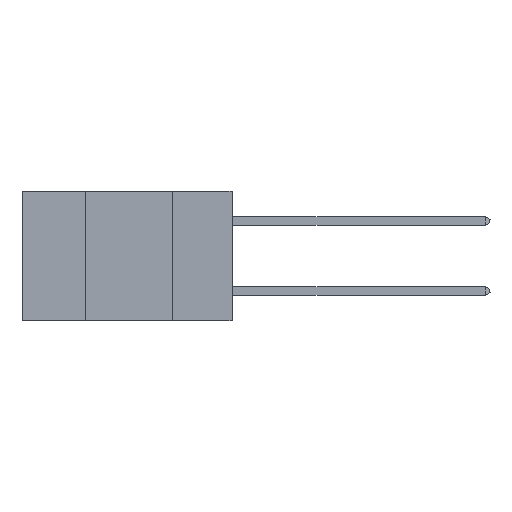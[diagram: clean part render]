
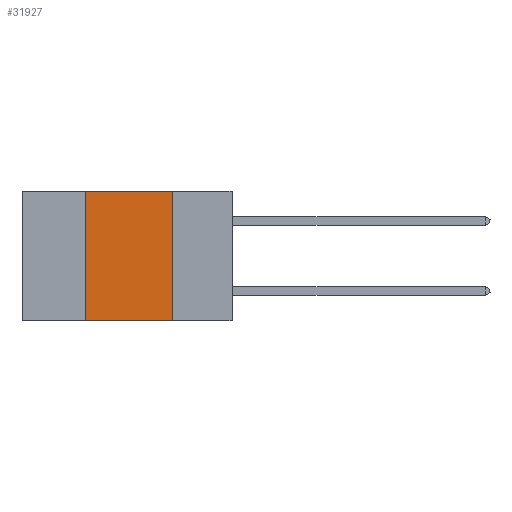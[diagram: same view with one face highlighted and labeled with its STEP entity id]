
A CAD part, left-side view. The second image highlights one B-rep face of the part: STEP entity #31927.
In plain terms, the highlighted planar face has unit normal (-1, 0, 0).
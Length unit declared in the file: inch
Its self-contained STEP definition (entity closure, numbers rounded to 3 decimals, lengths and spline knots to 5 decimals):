
#626 = LINE ( 'NONE', #4560, #36915 ) ;
#800 = VERTEX_POINT ( 'NONE', #27036 ) ;
#1800 = CARTESIAN_POINT ( 'NONE',  ( 0., 0.6, -0.37 ) ) ;
#3225 = ORIENTED_EDGE ( 'NONE', *, *, #5137, .F. ) ;
#3262 = LINE ( 'NONE', #1800, #23564 ) ;
#4131 = DIRECTION ( 'NONE',  ( 1., 0., 0. ) ) ;
#4560 = CARTESIAN_POINT ( 'NONE',  ( 0., 0.6, 0. ) ) ;
#5137 = EDGE_CURVE ( 'NONE', #35858, #800, #36840, .T. ) ;
#9967 = DIRECTION ( 'NONE',  ( 0., 0., -1. ) ) ;
#11135 = ORIENTED_EDGE ( 'NONE', *, *, #39826, .T. ) ;
#15299 = VERTEX_POINT ( 'NONE', #17003 ) ;
#16787 = CARTESIAN_POINT ( 'NONE',  ( 0., 0.17, 0. ) ) ;
#17003 = CARTESIAN_POINT ( 'NONE',  ( 0., 0.42, -0.37 ) ) ;
#17058 = CARTESIAN_POINT ( 'NONE',  ( 0., 0.42, 0. ) ) ;
#21544 = DIRECTION ( 'NONE',  ( 0., 0., -1. ) ) ;
#21793 = EDGE_CURVE ( 'NONE', #42769, #35858, #626, .T. ) ;
#23564 = VECTOR ( 'NONE', #42945, 39.37008 ) ;
#24684 = CARTESIAN_POINT ( 'NONE',  ( 0., 0.6, 0. ) ) ;
#26391 = CARTESIAN_POINT ( 'NONE',  ( 0., 0.42, 0. ) ) ;
#27036 = CARTESIAN_POINT ( 'NONE',  ( 0., 0.17, -0.37 ) ) ;
#29459 = VECTOR ( 'NONE', #33822, 39.37008 ) ;
#29962 = VECTOR ( 'NONE', #9967, 39.37008 ) ;
#31508 = ORIENTED_EDGE ( 'NONE', *, *, #37702, .F. ) ;
#31665 = PLANE ( 'NONE',  #40323 ) ;
#31927 = ADVANCED_FACE ( 'NONE', ( #39287 ), #31665, .F. ) ;
#33002 = CARTESIAN_POINT ( 'NONE',  ( 0., 0.17, 0. ) ) ;
#33822 = DIRECTION ( 'NONE',  ( 0., 0., 1. ) ) ;
#34938 = DIRECTION ( 'NONE',  ( 0., -1., 0. ) ) ;
#35858 = VERTEX_POINT ( 'NONE', #33002 ) ;
#36725 = EDGE_LOOP ( 'NONE', ( #3225, #41319, #31508, #11135 ) ) ;
#36840 = LINE ( 'NONE', #16787, #29962 ) ;
#36915 = VECTOR ( 'NONE', #34938, 39.37008 ) ;
#37702 = EDGE_CURVE ( 'NONE', #15299, #42769, #41719, .T. ) ;
#39287 = FACE_OUTER_BOUND ( 'NONE', #36725, .T. ) ;
#39826 = EDGE_CURVE ( 'NONE', #15299, #800, #3262, .T. ) ;
#40323 = AXIS2_PLACEMENT_3D ( 'NONE', #24684, #4131, #21544 ) ;
#41319 = ORIENTED_EDGE ( 'NONE', *, *, #21793, .F. ) ;
#41719 = LINE ( 'NONE', #26391, #29459 ) ;
#42769 = VERTEX_POINT ( 'NONE', #17058 ) ;
#42945 = DIRECTION ( 'NONE',  ( 0., -1., 0. ) ) ;
